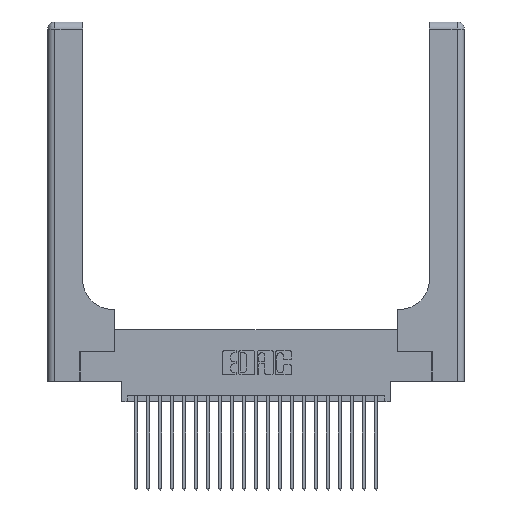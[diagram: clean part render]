
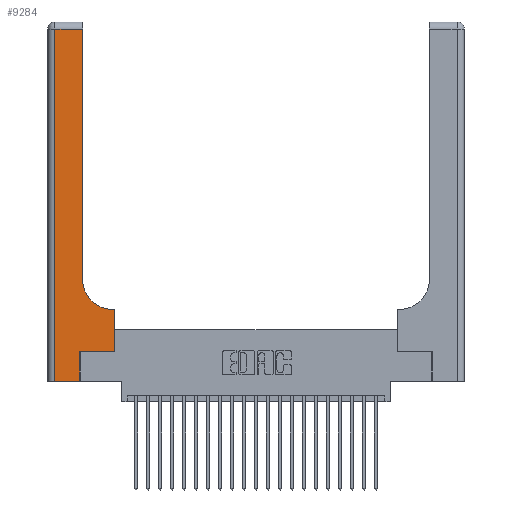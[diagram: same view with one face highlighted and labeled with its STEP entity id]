
A CAD part, top view. The second image highlights one B-rep face of the part: STEP entity #9284.
In plain terms, the highlighted planar face has unit normal (0, 0, 1).
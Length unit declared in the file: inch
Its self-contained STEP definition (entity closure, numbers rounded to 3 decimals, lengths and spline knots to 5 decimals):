
#63 = CARTESIAN_POINT ( 'NONE',  ( 0.269, 0., 0.37 ) ) ;
#159 = CARTESIAN_POINT ( 'NONE',  ( 0., 3., 0.37 ) ) ;
#234 = EDGE_LOOP ( 'NONE', ( #22836, #11675, #11578, #19326, #20478, #17841, #10530, #14414, #18823 ) ) ;
#669 = CARTESIAN_POINT ( 'NONE',  ( 0.06, 2.94, 0.37 ) ) ;
#772 = VERTEX_POINT ( 'NONE', #21904 ) ;
#849 = DIRECTION ( 'NONE',  ( 0., 0., -1. ) ) ;
#964 = DIRECTION ( 'NONE',  ( 0., 1., 0. ) ) ;
#1631 = VERTEX_POINT ( 'NONE', #7675 ) ;
#1722 = EDGE_CURVE ( 'NONE', #19319, #17923, #21277, .T. ) ;
#1927 = VERTEX_POINT ( 'NONE', #12377 ) ;
#2029 = DIRECTION ( 'NONE',  ( 0., 1., 0. ) ) ;
#2126 = DIRECTION ( 'NONE',  ( 0., 0., -1. ) ) ;
#2871 = EDGE_CURVE ( 'NONE', #1631, #1927, #18869, .T. ) ;
#2907 = CARTESIAN_POINT ( 'NONE',  ( 0.5585, 0.25, 0.37 ) ) ;
#3015 = EDGE_CURVE ( 'NONE', #17923, #16015, #5790, .T. ) ;
#4001 = VECTOR ( 'NONE', #6022, 39.37008 ) ;
#4074 = CARTESIAN_POINT ( 'NONE',  ( 0., 0., 0.37 ) ) ;
#4110 = CARTESIAN_POINT ( 'NONE',  ( 0.06, 3., 0.37 ) ) ;
#4687 = FACE_OUTER_BOUND ( 'NONE', #234, .T. ) ;
#5790 = LINE ( 'NONE', #63, #15935 ) ;
#6022 = DIRECTION ( 'NONE',  ( 0., -1., 0. ) ) ;
#6123 = VECTOR ( 'NONE', #19181, 39.37008 ) ;
#6369 = EDGE_CURVE ( 'NONE', #16891, #1631, #24063, .T. ) ;
#7287 = CARTESIAN_POINT ( 'NONE',  ( 0.2915, 0.6, 0.37 ) ) ;
#7323 = VECTOR ( 'NONE', #7670, 39.37008 ) ;
#7670 = DIRECTION ( 'NONE',  ( 1., 0., 0. ) ) ;
#7675 = CARTESIAN_POINT ( 'NONE',  ( 0.2915, 0.85, 0.37 ) ) ;
#8219 = CARTESIAN_POINT ( 'NONE',  ( 0.269, 0.25, 0.37 ) ) ;
#8716 = VECTOR ( 'NONE', #22764, 39.37008 ) ;
#8763 = VECTOR ( 'NONE', #964, 39.37008 ) ;
#9123 = LINE ( 'NONE', #4110, #4001 ) ;
#9238 = DIRECTION ( 'NONE',  ( 0., 1., 0. ) ) ;
#9284 = ADVANCED_FACE ( 'NONE', ( #4687 ), #11667, .F. ) ;
#10530 = ORIENTED_EDGE ( 'NONE', *, *, #22898, .T. ) ;
#10786 = CARTESIAN_POINT ( 'NONE',  ( 0.06, 0., 0.37 ) ) ;
#10811 = VERTEX_POINT ( 'NONE', #10855 ) ;
#10855 = CARTESIAN_POINT ( 'NONE',  ( 0.5585, 0.25, 0.37 ) ) ;
#11220 = EDGE_CURVE ( 'NONE', #11352, #19319, #9123, .T. ) ;
#11352 = VERTEX_POINT ( 'NONE', #669 ) ;
#11578 = ORIENTED_EDGE ( 'NONE', *, *, #11220, .T. ) ;
#11667 = PLANE ( 'NONE',  #14404 ) ;
#11675 = ORIENTED_EDGE ( 'NONE', *, *, #23841, .T. ) ;
#11812 = AXIS2_PLACEMENT_3D ( 'NONE', #12341, #849, #14250 ) ;
#12341 = CARTESIAN_POINT ( 'NONE',  ( 0.5415, 0.85, 0.37 ) ) ;
#12377 = CARTESIAN_POINT ( 'NONE',  ( 0.2915, 2.94, 0.37 ) ) ;
#13178 = VECTOR ( 'NONE', #24394, 39.37008 ) ;
#13848 = LINE ( 'NONE', #2907, #8763 ) ;
#14250 = DIRECTION ( 'NONE',  ( 1., 0., 0. ) ) ;
#14374 = LINE ( 'NONE', #7287, #13178 ) ;
#14404 = AXIS2_PLACEMENT_3D ( 'NONE', #159, #2126, #15455 ) ;
#14414 = ORIENTED_EDGE ( 'NONE', *, *, #24359, .T. ) ;
#14426 = CARTESIAN_POINT ( 'NONE',  ( 0.269, 0., 0.37 ) ) ;
#15022 = CARTESIAN_POINT ( 'NONE',  ( 0.5415, 0.6, 0.37 ) ) ;
#15455 = DIRECTION ( 'NONE',  ( -1., 0., 0. ) ) ;
#15935 = VECTOR ( 'NONE', #2029, 39.37008 ) ;
#16015 = VERTEX_POINT ( 'NONE', #8219 ) ;
#16891 = VERTEX_POINT ( 'NONE', #15022 ) ;
#17841 = ORIENTED_EDGE ( 'NONE', *, *, #20780, .T. ) ;
#17923 = VERTEX_POINT ( 'NONE', #14426 ) ;
#18275 = VECTOR ( 'NONE', #9238, 39.37008 ) ;
#18823 = ORIENTED_EDGE ( 'NONE', *, *, #6369, .T. ) ;
#18869 = LINE ( 'NONE', #22476, #18275 ) ;
#19018 = CARTESIAN_POINT ( 'NONE',  ( 0.269, 0.25, 0.37 ) ) ;
#19181 = DIRECTION ( 'NONE',  ( 1., 0., 0. ) ) ;
#19319 = VERTEX_POINT ( 'NONE', #10786 ) ;
#19326 = ORIENTED_EDGE ( 'NONE', *, *, #1722, .T. ) ;
#20478 = ORIENTED_EDGE ( 'NONE', *, *, #3015, .T. ) ;
#20780 = EDGE_CURVE ( 'NONE', #16015, #10811, #21273, .T. ) ;
#21273 = LINE ( 'NONE', #19018, #7323 ) ;
#21277 = LINE ( 'NONE', #4074, #6123 ) ;
#21904 = CARTESIAN_POINT ( 'NONE',  ( 0.5585, 0.6, 0.37 ) ) ;
#22476 = CARTESIAN_POINT ( 'NONE',  ( 0.2915, 3., 0.37 ) ) ;
#22764 = DIRECTION ( 'NONE',  ( -1., 0., 0. ) ) ;
#22836 = ORIENTED_EDGE ( 'NONE', *, *, #2871, .T. ) ;
#22898 = EDGE_CURVE ( 'NONE', #10811, #772, #13848, .T. ) ;
#23824 = LINE ( 'NONE', #24662, #8716 ) ;
#23841 = EDGE_CURVE ( 'NONE', #1927, #11352, #23824, .T. ) ;
#24063 = CIRCLE ( 'NONE', #11812, 0.25 ) ;
#24359 = EDGE_CURVE ( 'NONE', #772, #16891, #14374, .T. ) ;
#24394 = DIRECTION ( 'NONE',  ( -1., 0., 0. ) ) ;
#24662 = CARTESIAN_POINT ( 'NONE',  ( 0., 2.94, 0.37 ) ) ;
